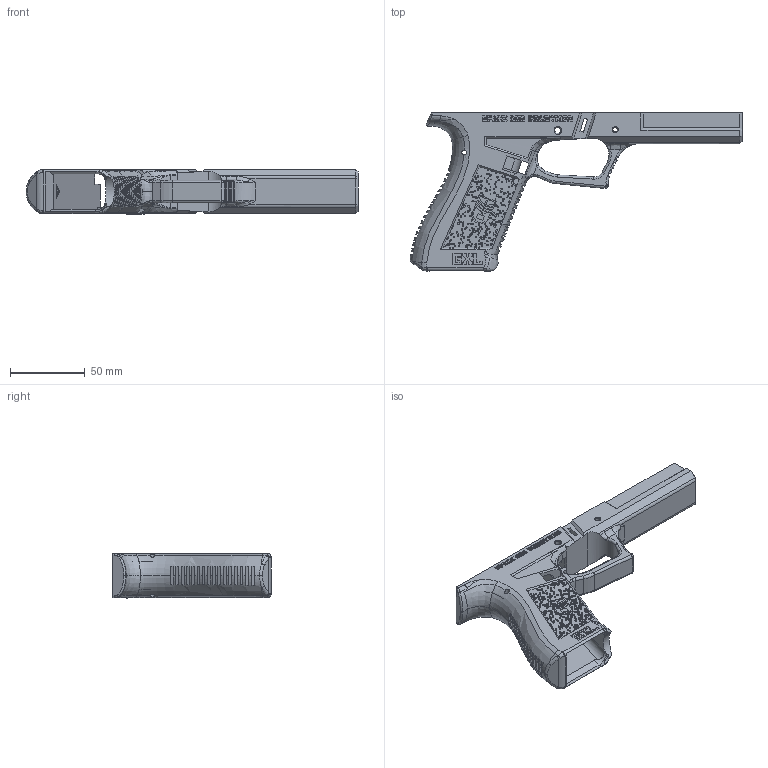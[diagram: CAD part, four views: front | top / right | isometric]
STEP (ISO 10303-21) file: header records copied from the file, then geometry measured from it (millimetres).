
FILE_DESCRIPTION(/* description */ (''),/* implementation_level */ '2;1');
FILE_NAME(/* name */ 'PY2A SDI GXL34.step',/* time_stamp */ '2022-06-24T22:01:37-05:00',/* author */ (''),/* organization */ (''),/* preprocessor_version */ 'ST-DEVELOPER v19',/* originating_system */ 'Autodesk Translation Framework v11.7.0.108',/* authorisation */ '');
FILE_SCHEMA (('AUTOMOTIVE_DESIGN { 1 0 10303 214 3 1 1 }'));
Products named in the file (1): PY2A SDI GXL/R
Bounding box: 221.76 x 105.56 x 29.73 mm (x, y, z)
Volume: 120350.5 mm3; surface area: 54643 mm2
Topology: 1 solids, 2 shells, 3554 faces, 9303 edges, 6153 vertices
Faces by surface type: bspline 2394, plane 1097, cylinder 54, torus 7, cone 2
Full cylindrical faces by diameter (mm): 1.933 x1, 3.05 x2, 3.146 x2, 3.5 x1, 4.1 x2
Entity records: 142607 total; most frequent: CARTESIAN_POINT 78560, ORIENTED_EDGE 18588, EDGE_CURVE 9294, DIRECTION 6635, VERTEX_POINT 6153, EDGE_LOOP 3989, LINE 3851, VECTOR 3851
